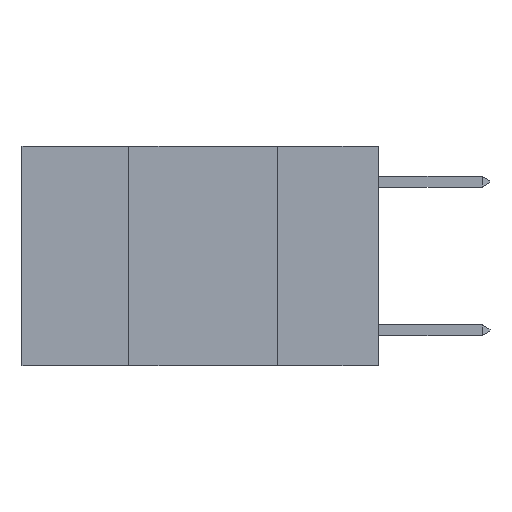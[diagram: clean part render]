
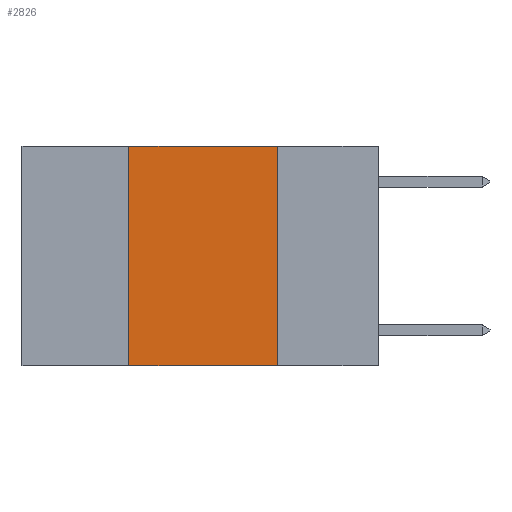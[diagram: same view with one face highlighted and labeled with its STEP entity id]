
A CAD part, left-side view. The second image highlights one B-rep face of the part: STEP entity #2826.
In plain terms, the highlighted planar face has unit normal (-1, 0, 0).
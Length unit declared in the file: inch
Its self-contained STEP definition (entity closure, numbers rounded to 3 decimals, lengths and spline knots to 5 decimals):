
#242 = EDGE_CURVE ( 'NONE', #8689, #1022, #10127, .T. ) ;
#645 = CARTESIAN_POINT ( 'NONE',  ( 0., 0.42, 0. ) ) ;
#729 = CARTESIAN_POINT ( 'NONE',  ( 0., 0.17, 0. ) ) ;
#822 = FACE_OUTER_BOUND ( 'NONE', #1938, .T. ) ;
#1004 = VERTEX_POINT ( 'NONE', #3412 ) ;
#1022 = VERTEX_POINT ( 'NONE', #8898 ) ;
#1938 = EDGE_LOOP ( 'NONE', ( #9280, #9428, #9584, #9858 ) ) ;
#2452 = CARTESIAN_POINT ( 'NONE',  ( 0., 0.6, -0.37 ) ) ;
#2595 = VECTOR ( 'NONE', #4585, 39.37008 ) ;
#2826 = ADVANCED_FACE ( 'NONE', ( #822 ), #6096, .F. ) ;
#3412 = CARTESIAN_POINT ( 'NONE',  ( 0., 0.17, 0. ) ) ;
#3617 = CARTESIAN_POINT ( 'NONE',  ( 0., 0.6, 0. ) ) ;
#3711 = VECTOR ( 'NONE', #4046, 39.37008 ) ;
#4046 = DIRECTION ( 'NONE',  ( 0., 0., 1. ) ) ;
#4247 = VECTOR ( 'NONE', #8497, 39.37008 ) ;
#4585 = DIRECTION ( 'NONE',  ( 0., -1., 0. ) ) ;
#5995 = DIRECTION ( 'NONE',  ( 0., 0., -1. ) ) ;
#6002 = CARTESIAN_POINT ( 'NONE',  ( 0., 0.42, -0.37 ) ) ;
#6017 = DIRECTION ( 'NONE',  ( 1., 0., 0. ) ) ;
#6030 = CARTESIAN_POINT ( 'NONE',  ( 0., 0.6, 0. ) ) ;
#6096 = PLANE ( 'NONE',  #10398 ) ;
#6710 = VERTEX_POINT ( 'NONE', #9723 ) ;
#7966 = EDGE_CURVE ( 'NONE', #1004, #6710, #8727, .T. ) ;
#7979 = EDGE_CURVE ( 'NONE', #8689, #6710, #10526, .T. ) ;
#8475 = VECTOR ( 'NONE', #9344, 39.37008 ) ;
#8497 = DIRECTION ( 'NONE',  ( 0., 0., -1. ) ) ;
#8689 = VERTEX_POINT ( 'NONE', #6002 ) ;
#8727 = LINE ( 'NONE', #729, #4247 ) ;
#8898 = CARTESIAN_POINT ( 'NONE',  ( 0., 0.42, 0. ) ) ;
#8978 = EDGE_CURVE ( 'NONE', #1022, #1004, #9468, .T. ) ;
#9280 = ORIENTED_EDGE ( 'NONE', *, *, #7966, .F. ) ;
#9344 = DIRECTION ( 'NONE',  ( 0., -1., 0. ) ) ;
#9428 = ORIENTED_EDGE ( 'NONE', *, *, #8978, .F. ) ;
#9468 = LINE ( 'NONE', #3617, #2595 ) ;
#9584 = ORIENTED_EDGE ( 'NONE', *, *, #242, .F. ) ;
#9723 = CARTESIAN_POINT ( 'NONE',  ( 0., 0.17, -0.37 ) ) ;
#9858 = ORIENTED_EDGE ( 'NONE', *, *, #7979, .T. ) ;
#10127 = LINE ( 'NONE', #645, #3711 ) ;
#10398 = AXIS2_PLACEMENT_3D ( 'NONE', #6030, #6017, #5995 ) ;
#10526 = LINE ( 'NONE', #2452, #8475 ) ;
